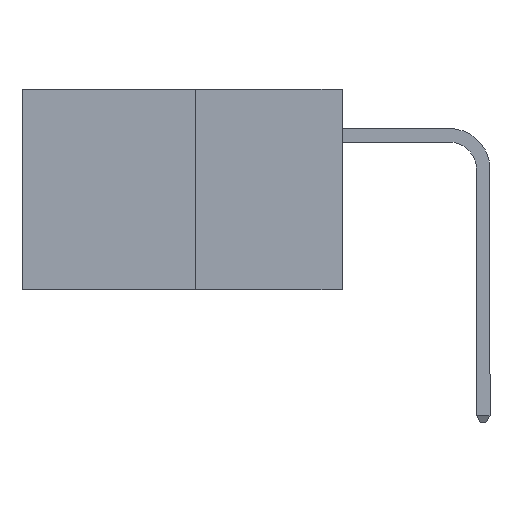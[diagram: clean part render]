
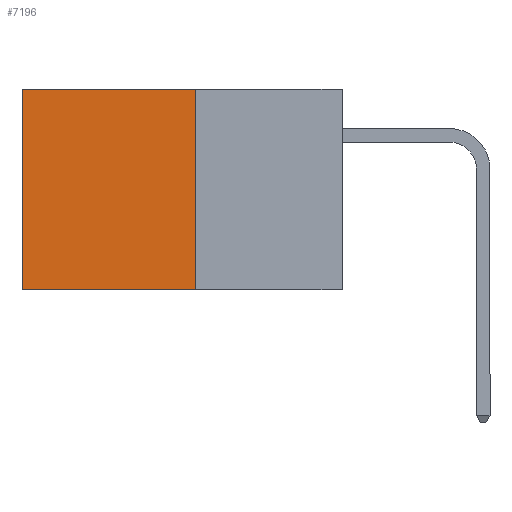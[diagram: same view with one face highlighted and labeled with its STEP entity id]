
A CAD part, left-side view. The second image highlights one B-rep face of the part: STEP entity #7196.
In plain terms, the highlighted planar face has unit normal (-1, 0, 0).
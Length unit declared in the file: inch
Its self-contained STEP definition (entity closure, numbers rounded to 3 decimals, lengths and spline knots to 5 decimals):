
#14 = CARTESIAN_POINT ( 'NONE',  ( 0.277, 0.59, 0. ) ) ;
#1185 = EDGE_CURVE ( 'NONE', #1357, #7241, #12065, .T. ) ;
#1357 = VERTEX_POINT ( 'NONE', #14 ) ;
#1960 = EDGE_CURVE ( 'NONE', #4572, #1357, #9873, .T. ) ;
#2194 = DIRECTION ( 'NONE',  ( 0., 0., -1. ) ) ;
#2530 = CARTESIAN_POINT ( 'NONE',  ( 0.277, 0.27, -0.37 ) ) ;
#2628 = EDGE_CURVE ( 'NONE', #4572, #9216, #10435, .T. ) ;
#3392 = VECTOR ( 'NONE', #6289, 39.37008 ) ;
#3978 = CARTESIAN_POINT ( 'NONE',  ( 0.277, 0.27, -0.37 ) ) ;
#4338 = VECTOR ( 'NONE', #11624, 39.37008 ) ;
#4572 = VERTEX_POINT ( 'NONE', #15927 ) ;
#5369 = EDGE_CURVE ( 'NONE', #9216, #7241, #14315, .T. ) ;
#6152 = ORIENTED_EDGE ( 'NONE', *, *, #1185, .T. ) ;
#6171 = ORIENTED_EDGE ( 'NONE', *, *, #5369, .F. ) ;
#6193 = VECTOR ( 'NONE', #2194, 39.37008 ) ;
#6217 = AXIS2_PLACEMENT_3D ( 'NONE', #8095, #7969, #7915 ) ;
#6277 = ORIENTED_EDGE ( 'NONE', *, *, #2628, .F. ) ;
#6289 = DIRECTION ( 'NONE',  ( 0., 0., -1. ) ) ;
#6339 = EDGE_LOOP ( 'NONE', ( #6152, #6171, #6277, #6447 ) ) ;
#6447 = ORIENTED_EDGE ( 'NONE', *, *, #1960, .T. ) ;
#6543 = VECTOR ( 'NONE', #13969, 39.37008 ) ;
#6955 = CARTESIAN_POINT ( 'NONE',  ( 0.277, 0.59, -0.37 ) ) ;
#7196 = ADVANCED_FACE ( 'NONE', ( #8186 ), #8166, .F. ) ;
#7241 = VERTEX_POINT ( 'NONE', #7272 ) ;
#7272 = CARTESIAN_POINT ( 'NONE',  ( 0.277, 0.59, -0.37 ) ) ;
#7915 = DIRECTION ( 'NONE',  ( 0., 0., -1. ) ) ;
#7969 = DIRECTION ( 'NONE',  ( 1., 0., 0. ) ) ;
#8095 = CARTESIAN_POINT ( 'NONE',  ( 0.277, 0.27, -0.37 ) ) ;
#8166 = PLANE ( 'NONE',  #6217 ) ;
#8186 = FACE_OUTER_BOUND ( 'NONE', #6339, .T. ) ;
#9216 = VERTEX_POINT ( 'NONE', #2530 ) ;
#9873 = LINE ( 'NONE', #11307, #6543 ) ;
#10435 = LINE ( 'NONE', #3978, #3392 ) ;
#11307 = CARTESIAN_POINT ( 'NONE',  ( 0.277, 0.27, 0. ) ) ;
#11624 = DIRECTION ( 'NONE',  ( 0., 1., 0. ) ) ;
#12065 = LINE ( 'NONE', #6955, #6193 ) ;
#12159 = CARTESIAN_POINT ( 'NONE',  ( 0.277, 0.27, -0.37 ) ) ;
#13969 = DIRECTION ( 'NONE',  ( 0., 1., 0. ) ) ;
#14315 = LINE ( 'NONE', #12159, #4338 ) ;
#15927 = CARTESIAN_POINT ( 'NONE',  ( 0.277, 0.27, 0. ) ) ;
